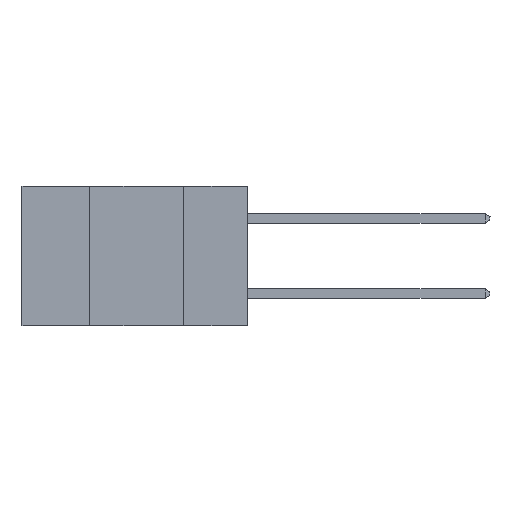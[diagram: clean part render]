
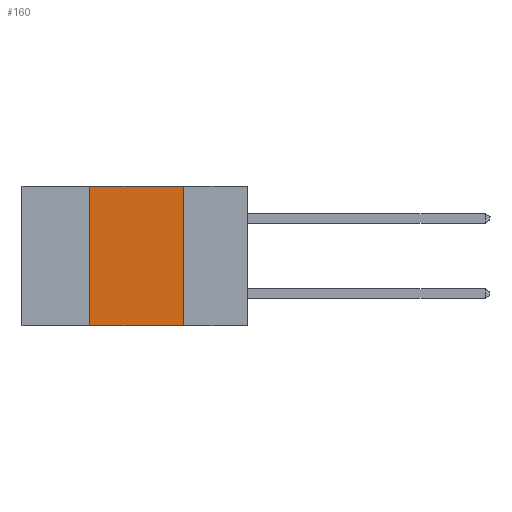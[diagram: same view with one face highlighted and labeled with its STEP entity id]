
A CAD part, left-side view. The second image highlights one B-rep face of the part: STEP entity #160.
In plain terms, the highlighted planar face has unit normal (-1, 0, 0).
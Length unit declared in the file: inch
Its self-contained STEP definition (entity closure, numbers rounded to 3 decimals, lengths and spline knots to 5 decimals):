
#160 = ADVANCED_FACE ( 'NONE', ( #4371 ), #622, .F. ) ;
#622 = PLANE ( 'NONE',  #2918 ) ;
#1847 = DIRECTION ( 'NONE',  ( 0., 0., -1. ) ) ;
#1865 = VERTEX_POINT ( 'NONE', #24596 ) ;
#2219 = CARTESIAN_POINT ( 'NONE',  ( 0., 0.42, -0.37 ) ) ;
#2918 = AXIS2_PLACEMENT_3D ( 'NONE', #19214, #11853, #8213 ) ;
#4371 = FACE_OUTER_BOUND ( 'NONE', #18759, .T. ) ;
#4697 = DIRECTION ( 'NONE',  ( 0., -1., 0. ) ) ;
#5729 = ORIENTED_EDGE ( 'NONE', *, *, #16591, .T. ) ;
#7319 = ORIENTED_EDGE ( 'NONE', *, *, #17397, .F. ) ;
#8213 = DIRECTION ( 'NONE',  ( 0., 0., -1. ) ) ;
#8265 = CARTESIAN_POINT ( 'NONE',  ( 0., 0.42, 0. ) ) ;
#8275 = VECTOR ( 'NONE', #1847, 39.37008 ) ;
#9113 = VECTOR ( 'NONE', #19324, 39.37008 ) ;
#10180 = LINE ( 'NONE', #10311, #19061 ) ;
#10311 = CARTESIAN_POINT ( 'NONE',  ( 0., 0.6, -0.37 ) ) ;
#10558 = VERTEX_POINT ( 'NONE', #23535 ) ;
#11666 = EDGE_CURVE ( 'NONE', #20340, #1865, #13692, .T. ) ;
#11829 = DIRECTION ( 'NONE',  ( 0., -1., 0. ) ) ;
#11853 = DIRECTION ( 'NONE',  ( 1., 0., 0. ) ) ;
#12106 = VERTEX_POINT ( 'NONE', #2219 ) ;
#13692 = LINE ( 'NONE', #16874, #16284 ) ;
#14254 = ORIENTED_EDGE ( 'NONE', *, *, #17840, .F. ) ;
#14877 = LINE ( 'NONE', #23062, #9113 ) ;
#15196 = LINE ( 'NONE', #22664, #8275 ) ;
#16284 = VECTOR ( 'NONE', #11829, 39.37008 ) ;
#16591 = EDGE_CURVE ( 'NONE', #12106, #10558, #10180, .T. ) ;
#16874 = CARTESIAN_POINT ( 'NONE',  ( 0., 0.6, 0. ) ) ;
#17397 = EDGE_CURVE ( 'NONE', #12106, #20340, #14877, .T. ) ;
#17840 = EDGE_CURVE ( 'NONE', #1865, #10558, #15196, .T. ) ;
#18759 = EDGE_LOOP ( 'NONE', ( #14254, #19857, #7319, #5729 ) ) ;
#19061 = VECTOR ( 'NONE', #4697, 39.37008 ) ;
#19214 = CARTESIAN_POINT ( 'NONE',  ( 0., 0.6, 0. ) ) ;
#19324 = DIRECTION ( 'NONE',  ( 0., 0., 1. ) ) ;
#19857 = ORIENTED_EDGE ( 'NONE', *, *, #11666, .F. ) ;
#20340 = VERTEX_POINT ( 'NONE', #8265 ) ;
#22664 = CARTESIAN_POINT ( 'NONE',  ( 0., 0.17, -0.37 ) ) ;
#23062 = CARTESIAN_POINT ( 'NONE',  ( 0., 0.42, -0.37 ) ) ;
#23535 = CARTESIAN_POINT ( 'NONE',  ( 0., 0.17, -0.37 ) ) ;
#24596 = CARTESIAN_POINT ( 'NONE',  ( 0., 0.17, 0. ) ) ;
